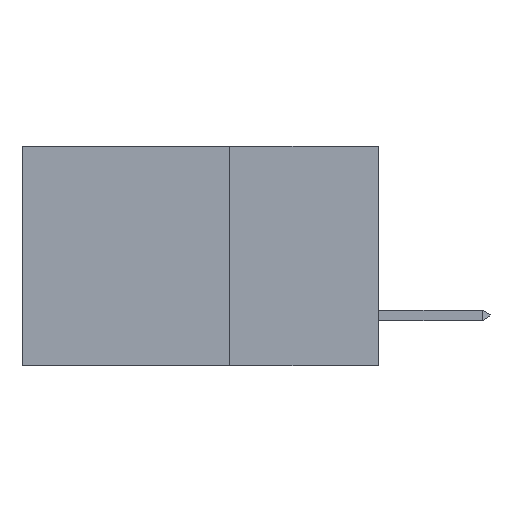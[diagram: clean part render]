
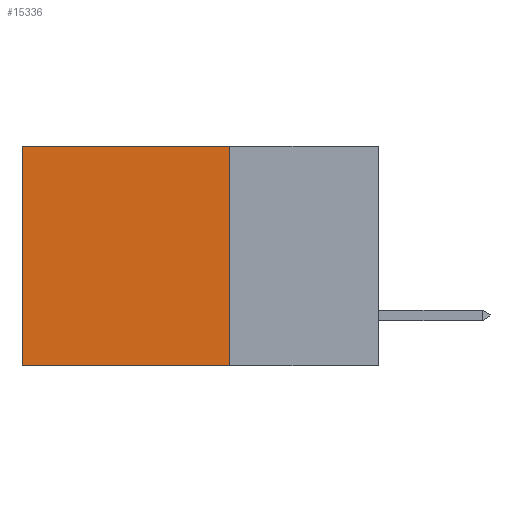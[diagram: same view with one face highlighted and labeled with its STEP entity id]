
A CAD part, left-side view. The second image highlights one B-rep face of the part: STEP entity #15336.
In plain terms, the highlighted planar face has unit normal (-1, 0, 0).
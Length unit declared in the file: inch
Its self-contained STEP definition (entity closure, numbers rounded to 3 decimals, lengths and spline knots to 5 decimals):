
#639 = LINE ( 'NONE', #7829, #14391 ) ;
#1436 = AXIS2_PLACEMENT_3D ( 'NONE', #20444, #11163, #16972 ) ;
#2180 = DIRECTION ( 'NONE',  ( 0., 0., -1. ) ) ;
#2432 = CARTESIAN_POINT ( 'NONE',  ( 0.2615, 0.25, -0.37 ) ) ;
#3231 = CARTESIAN_POINT ( 'NONE',  ( 0.2615, 0.6, -0.37 ) ) ;
#3685 = CARTESIAN_POINT ( 'NONE',  ( 0.2615, 0.25, 0. ) ) ;
#5196 = CARTESIAN_POINT ( 'NONE',  ( 0.2615, 0.25, -0.37 ) ) ;
#5746 = PLANE ( 'NONE',  #1436 ) ;
#6309 = CARTESIAN_POINT ( 'NONE',  ( 0.2615, 0.25, -0.37 ) ) ;
#6959 = ORIENTED_EDGE ( 'NONE', *, *, #18466, .T. ) ;
#7287 = VERTEX_POINT ( 'NONE', #6309 ) ;
#7829 = CARTESIAN_POINT ( 'NONE',  ( 0.2615, 0.25, 0. ) ) ;
#8793 = VERTEX_POINT ( 'NONE', #3231 ) ;
#10453 = LINE ( 'NONE', #5196, #16144 ) ;
#10773 = LINE ( 'NONE', #14634, #14232 ) ;
#11163 = DIRECTION ( 'NONE',  ( 1., 0., 0. ) ) ;
#11973 = ORIENTED_EDGE ( 'NONE', *, *, #22224, .F. ) ;
#12190 = VECTOR ( 'NONE', #20564, 39.37008 ) ;
#12566 = DIRECTION ( 'NONE',  ( 0., 0., -1. ) ) ;
#13142 = LINE ( 'NONE', #2432, #12190 ) ;
#13943 = EDGE_LOOP ( 'NONE', ( #6959, #11973, #20690, #21592 ) ) ;
#14232 = VECTOR ( 'NONE', #2180, 39.37008 ) ;
#14391 = VECTOR ( 'NONE', #14995, 39.37008 ) ;
#14634 = CARTESIAN_POINT ( 'NONE',  ( 0.2615, 0.6, -0.37 ) ) ;
#14995 = DIRECTION ( 'NONE',  ( 0., 1., 0. ) ) ;
#15336 = ADVANCED_FACE ( 'NONE', ( #18520 ), #5746, .F. ) ;
#16144 = VECTOR ( 'NONE', #12566, 39.37008 ) ;
#16972 = DIRECTION ( 'NONE',  ( 0., 0., -1. ) ) ;
#18057 = EDGE_CURVE ( 'NONE', #20403, #7287, #10453, .T. ) ;
#18466 = EDGE_CURVE ( 'NONE', #20735, #8793, #10773, .T. ) ;
#18520 = FACE_OUTER_BOUND ( 'NONE', #13943, .T. ) ;
#20403 = VERTEX_POINT ( 'NONE', #3685 ) ;
#20444 = CARTESIAN_POINT ( 'NONE',  ( 0.2615, 0.25, -0.37 ) ) ;
#20564 = DIRECTION ( 'NONE',  ( 0., 1., 0. ) ) ;
#20690 = ORIENTED_EDGE ( 'NONE', *, *, #18057, .F. ) ;
#20735 = VERTEX_POINT ( 'NONE', #20987 ) ;
#20987 = CARTESIAN_POINT ( 'NONE',  ( 0.2615, 0.6, 0. ) ) ;
#21447 = EDGE_CURVE ( 'NONE', #20403, #20735, #639, .T. ) ;
#21592 = ORIENTED_EDGE ( 'NONE', *, *, #21447, .T. ) ;
#22224 = EDGE_CURVE ( 'NONE', #7287, #8793, #13142, .T. ) ;
